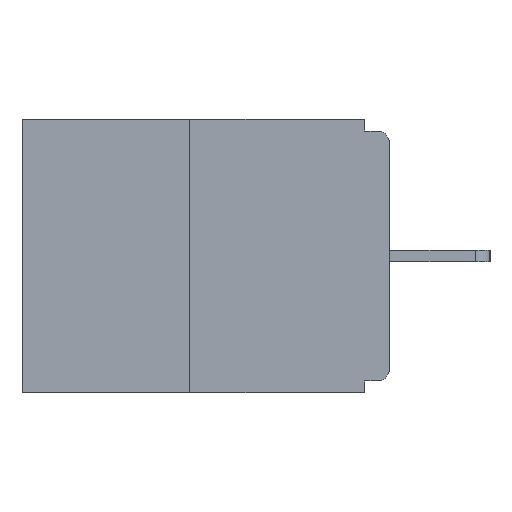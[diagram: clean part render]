
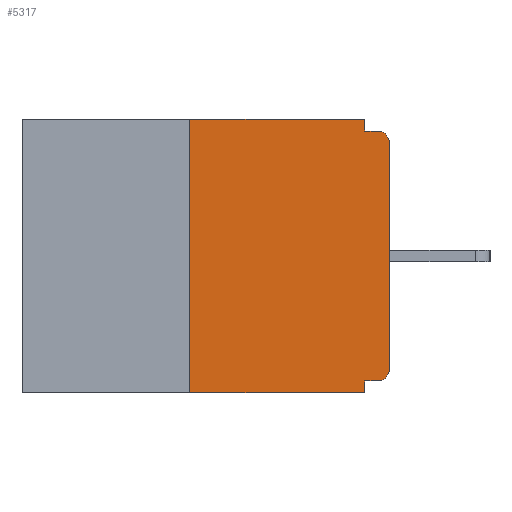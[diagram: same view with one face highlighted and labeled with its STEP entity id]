
A CAD part, left-side view. The second image highlights one B-rep face of the part: STEP entity #5317.
In plain terms, the highlighted planar face has unit normal (-1, 0, 0).
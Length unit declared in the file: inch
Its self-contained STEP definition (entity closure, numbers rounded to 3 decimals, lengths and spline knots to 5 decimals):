
#96 = CARTESIAN_POINT ( 'NONE',  ( 0., 0., -0.313 ) ) ;
#276 = ORIENTED_EDGE ( 'NONE', *, *, #6082, .F. ) ;
#585 = VERTEX_POINT ( 'NONE', #3172 ) ;
#1158 = LINE ( 'NONE', #2109, #10273 ) ;
#1194 = DIRECTION ( 'NONE',  ( 0., 1., 0. ) ) ;
#1368 = ORIENTED_EDGE ( 'NONE', *, *, #11282, .T. ) ;
#1439 = ORIENTED_EDGE ( 'NONE', *, *, #1723, .F. ) ;
#1460 = VERTEX_POINT ( 'NONE', #2112 ) ;
#1586 = CARTESIAN_POINT ( 'NONE',  ( 0., 0.031, -0.343 ) ) ;
#1723 = EDGE_CURVE ( 'NONE', #13550, #7230, #6672, .T. ) ;
#1817 = DIRECTION ( 'NONE',  ( -1., 0., 0. ) ) ;
#1876 = CARTESIAN_POINT ( 'NONE',  ( 0., 0., 0. ) ) ;
#2072 = LINE ( 'NONE', #4132, #10265 ) ;
#2109 = CARTESIAN_POINT ( 'NONE',  ( 0., 0., -0.015 ) ) ;
#2112 = CARTESIAN_POINT ( 'NONE',  ( 0., 0.031, -0.328 ) ) ;
#2230 = CARTESIAN_POINT ( 'NONE',  ( 0., 0.031, 0. ) ) ;
#2440 = VERTEX_POINT ( 'NONE', #4388 ) ;
#2475 = DIRECTION ( 'NONE',  ( 0., 0., -1. ) ) ;
#2615 = DIRECTION ( 'NONE',  ( 1., 0., 0. ) ) ;
#2797 = EDGE_CURVE ( 'NONE', #10026, #4083, #1158, .T. ) ;
#2812 = EDGE_LOOP ( 'NONE', ( #1439, #12597, #9745, #11740, #276, #1368, #5597, #5680, #11240, #7762 ) ) ;
#2879 = CARTESIAN_POINT ( 'NONE',  ( 0., 0.46, -0.343 ) ) ;
#2901 = VECTOR ( 'NONE', #10782, 39.37008 ) ;
#3172 = CARTESIAN_POINT ( 'NONE',  ( 0., 0., -0.03 ) ) ;
#3370 = CIRCLE ( 'NONE', #9405, 0.015 ) ;
#3478 = EDGE_CURVE ( 'NONE', #7230, #10026, #7517, .T. ) ;
#3549 = FACE_OUTER_BOUND ( 'NONE', #2812, .T. ) ;
#3607 = CARTESIAN_POINT ( 'NONE',  ( 0., 0.25, 0. ) ) ;
#3742 = CARTESIAN_POINT ( 'NONE',  ( 0., 0.015, -0.015 ) ) ;
#3825 = AXIS2_PLACEMENT_3D ( 'NONE', #12091, #2615, #2475 ) ;
#3923 = DIRECTION ( 'NONE',  ( 0., 0., 1. ) ) ;
#4083 = VERTEX_POINT ( 'NONE', #3742 ) ;
#4132 = CARTESIAN_POINT ( 'NONE',  ( 0., 0.25, 0. ) ) ;
#4388 = CARTESIAN_POINT ( 'NONE',  ( 0., 0.25, -0.343 ) ) ;
#5049 = LINE ( 'NONE', #1876, #12343 ) ;
#5230 = VERTEX_POINT ( 'NONE', #1586 ) ;
#5317 = ADVANCED_FACE ( 'NONE', ( #3549 ), #7839, .F. ) ;
#5407 = VECTOR ( 'NONE', #9552, 39.37008 ) ;
#5510 = CARTESIAN_POINT ( 'NONE',  ( 0., 0.031, -0.343 ) ) ;
#5597 = ORIENTED_EDGE ( 'NONE', *, *, #12307, .T. ) ;
#5680 = ORIENTED_EDGE ( 'NONE', *, *, #11205, .T. ) ;
#5917 = LINE ( 'NONE', #2879, #11304 ) ;
#6082 = EDGE_CURVE ( 'NONE', #9869, #1460, #6462, .T. ) ;
#6246 = DIRECTION ( 'NONE',  ( 0., 0., -1. ) ) ;
#6462 = LINE ( 'NONE', #10718, #10545 ) ;
#6494 = DIRECTION ( 'NONE',  ( 0., -1., 0. ) ) ;
#6672 = LINE ( 'NONE', #8819, #8880 ) ;
#6803 = VERTEX_POINT ( 'NONE', #96 ) ;
#6990 = CARTESIAN_POINT ( 'NONE',  ( 0., 0.015, -0.328 ) ) ;
#7230 = VERTEX_POINT ( 'NONE', #2230 ) ;
#7512 = DIRECTION ( 'NONE',  ( 0., 0., -1. ) ) ;
#7517 = LINE ( 'NONE', #11696, #2901 ) ;
#7762 = ORIENTED_EDGE ( 'NONE', *, *, #3478, .F. ) ;
#7839 = PLANE ( 'NONE',  #3825 ) ;
#7853 = CIRCLE ( 'NONE', #9618, 0.015 ) ;
#7876 = DIRECTION ( 'NONE',  ( 0., -1., 0. ) ) ;
#8386 = DIRECTION ( 'NONE',  ( 0., 0., 1. ) ) ;
#8536 = CARTESIAN_POINT ( 'NONE',  ( 0., 0.015, -0.313 ) ) ;
#8640 = LINE ( 'NONE', #5510, #5407 ) ;
#8819 = CARTESIAN_POINT ( 'NONE',  ( 0., 0.46, 0. ) ) ;
#8880 = VECTOR ( 'NONE', #7876, 39.37008 ) ;
#9405 = AXIS2_PLACEMENT_3D ( 'NONE', #8536, #10779, #7512 ) ;
#9552 = DIRECTION ( 'NONE',  ( 0., 0., -1. ) ) ;
#9618 = AXIS2_PLACEMENT_3D ( 'NONE', #11410, #1817, #6246 ) ;
#9745 = ORIENTED_EDGE ( 'NONE', *, *, #13596, .T. ) ;
#9869 = VERTEX_POINT ( 'NONE', #6990 ) ;
#10026 = VERTEX_POINT ( 'NONE', #10774 ) ;
#10103 = EDGE_CURVE ( 'NONE', #2440, #13550, #2072, .T. ) ;
#10265 = VECTOR ( 'NONE', #8386, 39.37008 ) ;
#10273 = VECTOR ( 'NONE', #6494, 39.37008 ) ;
#10545 = VECTOR ( 'NONE', #1194, 39.37008 ) ;
#10718 = CARTESIAN_POINT ( 'NONE',  ( 0., 0., -0.328 ) ) ;
#10774 = CARTESIAN_POINT ( 'NONE',  ( 0., 0.031, -0.015 ) ) ;
#10779 = DIRECTION ( 'NONE',  ( -1., 0., 0. ) ) ;
#10782 = DIRECTION ( 'NONE',  ( 0., 0., -1. ) ) ;
#11205 = EDGE_CURVE ( 'NONE', #585, #4083, #7853, .T. ) ;
#11218 = DIRECTION ( 'NONE',  ( 0., -1., 0. ) ) ;
#11240 = ORIENTED_EDGE ( 'NONE', *, *, #2797, .F. ) ;
#11282 = EDGE_CURVE ( 'NONE', #9869, #6803, #3370, .T. ) ;
#11304 = VECTOR ( 'NONE', #11218, 39.37008 ) ;
#11410 = CARTESIAN_POINT ( 'NONE',  ( 0., 0.015, -0.03 ) ) ;
#11655 = EDGE_CURVE ( 'NONE', #1460, #5230, #8640, .T. ) ;
#11696 = CARTESIAN_POINT ( 'NONE',  ( 0., 0.031, 0. ) ) ;
#11740 = ORIENTED_EDGE ( 'NONE', *, *, #11655, .F. ) ;
#12091 = CARTESIAN_POINT ( 'NONE',  ( 0., 0.46, 0. ) ) ;
#12307 = EDGE_CURVE ( 'NONE', #6803, #585, #5049, .T. ) ;
#12343 = VECTOR ( 'NONE', #3923, 39.37008 ) ;
#12597 = ORIENTED_EDGE ( 'NONE', *, *, #10103, .F. ) ;
#13550 = VERTEX_POINT ( 'NONE', #3607 ) ;
#13596 = EDGE_CURVE ( 'NONE', #2440, #5230, #5917, .T. ) ;
